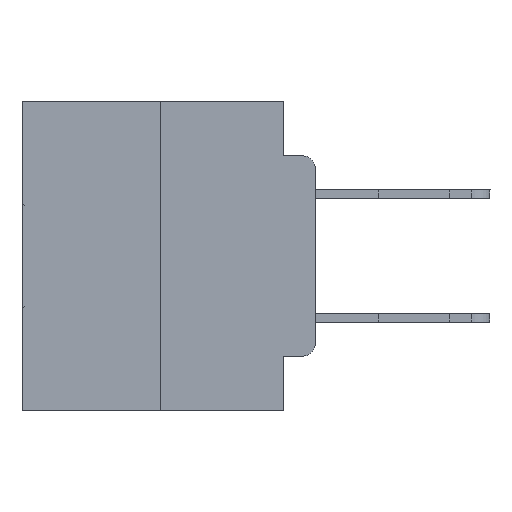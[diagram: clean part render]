
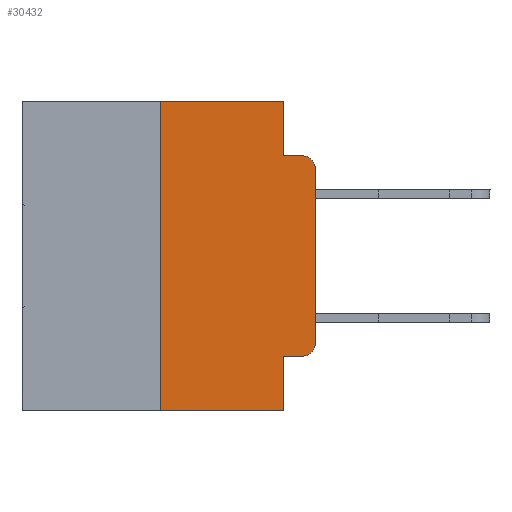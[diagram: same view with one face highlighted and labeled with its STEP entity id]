
A CAD part, left-side view. The second image highlights one B-rep face of the part: STEP entity #30432.
In plain terms, the highlighted planar face has unit normal (-1, 0, 0).
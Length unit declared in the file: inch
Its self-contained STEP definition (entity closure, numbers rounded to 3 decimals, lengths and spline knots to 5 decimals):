
#1 = LINE ( 'NONE', #14380, #24693 ) ;
#347 = VECTOR ( 'NONE', #18420, 39.37008 ) ;
#413 = CARTESIAN_POINT ( 'NONE',  ( 0., 0.051, 0. ) ) ;
#550 = CARTESIAN_POINT ( 'NONE',  ( 0., 0.02, -0.3915 ) ) ;
#879 = CIRCLE ( 'NONE', #11738, 0.02 ) ;
#952 = VERTEX_POINT ( 'NONE', #6747 ) ;
#1038 = DIRECTION ( 'NONE',  ( 0., -1., 0. ) ) ;
#1174 = VECTOR ( 'NONE', #9077, 39.37008 ) ;
#1950 = VECTOR ( 'NONE', #29991, 39.37008 ) ;
#2012 = CARTESIAN_POINT ( 'NONE',  ( 0., 0.02, -0.0885 ) ) ;
#2043 = LINE ( 'NONE', #9143, #347 ) ;
#2145 = LINE ( 'NONE', #20824, #6897 ) ;
#2231 = ORIENTED_EDGE ( 'NONE', *, *, #4443, .T. ) ;
#2256 = CARTESIAN_POINT ( 'NONE',  ( 0., 0.051, -0.5 ) ) ;
#2347 = AXIS2_PLACEMENT_3D ( 'NONE', #8305, #24803, #13262 ) ;
#3353 = ORIENTED_EDGE ( 'NONE', *, *, #26750, .T. ) ;
#3407 = EDGE_LOOP ( 'NONE', ( #3353, #2231, #6098, #15484, #16682, #26682, #7041, #8892, #13306, #4277 ) ) ;
#3780 = EDGE_CURVE ( 'NONE', #27124, #17725, #2043, .T. ) ;
#4271 = LINE ( 'NONE', #24948, #1950 ) ;
#4277 = ORIENTED_EDGE ( 'NONE', *, *, #9478, .T. ) ;
#4443 = EDGE_CURVE ( 'NONE', #952, #5365, #8770, .T. ) ;
#4929 = VERTEX_POINT ( 'NONE', #18425 ) ;
#5365 = VERTEX_POINT ( 'NONE', #2012 ) ;
#5950 = EDGE_CURVE ( 'NONE', #17725, #5365, #7191, .T. ) ;
#6098 = ORIENTED_EDGE ( 'NONE', *, *, #5950, .F. ) ;
#6747 = CARTESIAN_POINT ( 'NONE',  ( 0., 0., -0.1085 ) ) ;
#6795 = CARTESIAN_POINT ( 'NONE',  ( 0., 0.25, 0. ) ) ;
#6897 = VECTOR ( 'NONE', #16048, 39.37008 ) ;
#7041 = ORIENTED_EDGE ( 'NONE', *, *, #27512, .T. ) ;
#7191 = LINE ( 'NONE', #21097, #1174 ) ;
#7256 = DIRECTION ( 'NONE',  ( 0., 0., 1. ) ) ;
#8305 = CARTESIAN_POINT ( 'NONE',  ( 0., 0.02, -0.1085 ) ) ;
#8366 = CARTESIAN_POINT ( 'NONE',  ( 0., 0.051, -0.4115 ) ) ;
#8770 = CIRCLE ( 'NONE', #2347, 0.02 ) ;
#8823 = VECTOR ( 'NONE', #19301, 39.37008 ) ;
#8892 = ORIENTED_EDGE ( 'NONE', *, *, #12961, .F. ) ;
#9077 = DIRECTION ( 'NONE',  ( 0., -1., 0. ) ) ;
#9143 = CARTESIAN_POINT ( 'NONE',  ( 0., 0.051, 0. ) ) ;
#9478 = EDGE_CURVE ( 'NONE', #21237, #17521, #879, .T. ) ;
#9542 = CARTESIAN_POINT ( 'NONE',  ( 0., 0.473, 0. ) ) ;
#9899 = LINE ( 'NONE', #12225, #8823 ) ;
#9989 = DIRECTION ( 'NONE',  ( -1., 0., 0. ) ) ;
#10285 = VERTEX_POINT ( 'NONE', #6795 ) ;
#11014 = EDGE_CURVE ( 'NONE', #10285, #27124, #13246, .T. ) ;
#11738 = AXIS2_PLACEMENT_3D ( 'NONE', #550, #9989, #19246 ) ;
#12098 = CARTESIAN_POINT ( 'NONE',  ( 0., 0.051, -0.4115 ) ) ;
#12225 = CARTESIAN_POINT ( 'NONE',  ( 0., 0., 0. ) ) ;
#12327 = VECTOR ( 'NONE', #14253, 39.37008 ) ;
#12961 = EDGE_CURVE ( 'NONE', #29764, #14738, #2145, .T. ) ;
#13246 = LINE ( 'NONE', #22171, #20136 ) ;
#13262 = DIRECTION ( 'NONE',  ( 0., 0., -1. ) ) ;
#13306 = ORIENTED_EDGE ( 'NONE', *, *, #29633, .T. ) ;
#13797 = EDGE_CURVE ( 'NONE', #4929, #10285, #1, .T. ) ;
#14253 = DIRECTION ( 'NONE',  ( 0., -1., 0. ) ) ;
#14380 = CARTESIAN_POINT ( 'NONE',  ( 0., 0.25, 0. ) ) ;
#14738 = VERTEX_POINT ( 'NONE', #2256 ) ;
#14883 = CARTESIAN_POINT ( 'NONE',  ( 0., 0.02, -0.4115 ) ) ;
#15484 = ORIENTED_EDGE ( 'NONE', *, *, #3780, .F. ) ;
#16048 = DIRECTION ( 'NONE',  ( 0., 0., -1. ) ) ;
#16342 = DIRECTION ( 'NONE',  ( 1., 0., 0. ) ) ;
#16682 = ORIENTED_EDGE ( 'NONE', *, *, #11014, .F. ) ;
#17521 = VERTEX_POINT ( 'NONE', #22570 ) ;
#17725 = VERTEX_POINT ( 'NONE', #17729 ) ;
#17729 = CARTESIAN_POINT ( 'NONE',  ( 0., 0.051, -0.0885 ) ) ;
#18420 = DIRECTION ( 'NONE',  ( 0., 0., -1. ) ) ;
#18425 = CARTESIAN_POINT ( 'NONE',  ( 0., 0.25, -0.5 ) ) ;
#18515 = PLANE ( 'NONE',  #22228 ) ;
#19103 = DIRECTION ( 'NONE',  ( 0., 0., -1. ) ) ;
#19246 = DIRECTION ( 'NONE',  ( 0., 0., -1. ) ) ;
#19301 = DIRECTION ( 'NONE',  ( 0., 0., 1. ) ) ;
#20136 = VECTOR ( 'NONE', #1038, 39.37008 ) ;
#20497 = FACE_OUTER_BOUND ( 'NONE', #3407, .T. ) ;
#20824 = CARTESIAN_POINT ( 'NONE',  ( 0., 0.051, 0. ) ) ;
#21097 = CARTESIAN_POINT ( 'NONE',  ( 0., 0.051, -0.0885 ) ) ;
#21237 = VERTEX_POINT ( 'NONE', #14883 ) ;
#22171 = CARTESIAN_POINT ( 'NONE',  ( 0., 0.473, 0. ) ) ;
#22228 = AXIS2_PLACEMENT_3D ( 'NONE', #9542, #16342, #19103 ) ;
#22570 = CARTESIAN_POINT ( 'NONE',  ( 0., 0., -0.3915 ) ) ;
#24693 = VECTOR ( 'NONE', #7256, 39.37008 ) ;
#24803 = DIRECTION ( 'NONE',  ( -1., 0., 0. ) ) ;
#24948 = CARTESIAN_POINT ( 'NONE',  ( 0., 0.473, -0.5 ) ) ;
#26682 = ORIENTED_EDGE ( 'NONE', *, *, #13797, .F. ) ;
#26750 = EDGE_CURVE ( 'NONE', #17521, #952, #9899, .T. ) ;
#27124 = VERTEX_POINT ( 'NONE', #413 ) ;
#27512 = EDGE_CURVE ( 'NONE', #4929, #14738, #4271, .T. ) ;
#28521 = LINE ( 'NONE', #12098, #12327 ) ;
#29633 = EDGE_CURVE ( 'NONE', #29764, #21237, #28521, .T. ) ;
#29764 = VERTEX_POINT ( 'NONE', #8366 ) ;
#29991 = DIRECTION ( 'NONE',  ( 0., -1., 0. ) ) ;
#30432 = ADVANCED_FACE ( 'NONE', ( #20497 ), #18515, .F. ) ;
